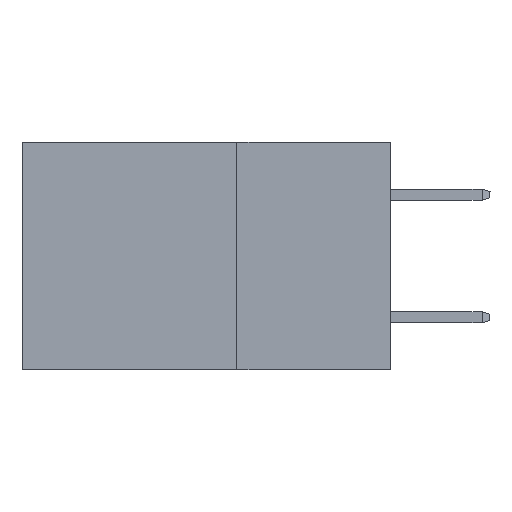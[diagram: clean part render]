
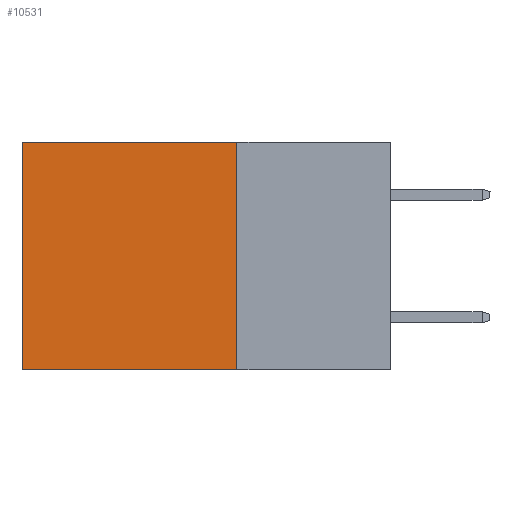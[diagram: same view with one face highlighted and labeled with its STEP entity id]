
A CAD part, left-side view. The second image highlights one B-rep face of the part: STEP entity #10531.
In plain terms, the highlighted planar face has unit normal (-1, 0, 0).
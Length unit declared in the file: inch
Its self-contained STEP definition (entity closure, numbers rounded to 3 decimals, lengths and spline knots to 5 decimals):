
#223 = DIRECTION ( 'NONE',  ( 0., 0., -1. ) ) ;
#842 = CARTESIAN_POINT ( 'NONE',  ( 0.2875, 0.25, 0. ) ) ;
#1834 = CARTESIAN_POINT ( 'NONE',  ( 0.2875, 0.25, -0.37 ) ) ;
#1917 = EDGE_CURVE ( 'NONE', #16710, #17223, #16675, .T. ) ;
#2002 = LINE ( 'NONE', #17564, #10388 ) ;
#2242 = DIRECTION ( 'NONE',  ( 1., 0., 0. ) ) ;
#2377 = VECTOR ( 'NONE', #4641, 39.37008 ) ;
#2421 = CARTESIAN_POINT ( 'NONE',  ( 0.2875, 0.25, 0. ) ) ;
#2541 = ORIENTED_EDGE ( 'NONE', *, *, #8119, .T. ) ;
#3652 = CARTESIAN_POINT ( 'NONE',  ( 0.2875, 0.25, 0. ) ) ;
#4612 = CARTESIAN_POINT ( 'NONE',  ( 0.2875, 0.6, -0.37 ) ) ;
#4641 = DIRECTION ( 'NONE',  ( 0., 1., 0. ) ) ;
#5062 = FACE_OUTER_BOUND ( 'NONE', #10837, .T. ) ;
#5237 = PLANE ( 'NONE',  #17324 ) ;
#5522 = ORIENTED_EDGE ( 'NONE', *, *, #15796, .F. ) ;
#5856 = LINE ( 'NONE', #8575, #2377 ) ;
#7149 = VERTEX_POINT ( 'NONE', #13517 ) ;
#7826 = DIRECTION ( 'NONE',  ( 0., 1., 0. ) ) ;
#8119 = EDGE_CURVE ( 'NONE', #7149, #11416, #2002, .T. ) ;
#8575 = CARTESIAN_POINT ( 'NONE',  ( 0.2875, 0.25, 0. ) ) ;
#9453 = DIRECTION ( 'NONE',  ( 0., 0., -1. ) ) ;
#10388 = VECTOR ( 'NONE', #223, 39.37008 ) ;
#10464 = CARTESIAN_POINT ( 'NONE',  ( 0.2875, 0.25, -0.37 ) ) ;
#10531 = ADVANCED_FACE ( 'NONE', ( #5062 ), #5237, .F. ) ;
#10837 = EDGE_LOOP ( 'NONE', ( #2541, #5522, #13476, #11723 ) ) ;
#11210 = EDGE_CURVE ( 'NONE', #16710, #7149, #5856, .T. ) ;
#11416 = VERTEX_POINT ( 'NONE', #4612 ) ;
#11723 = ORIENTED_EDGE ( 'NONE', *, *, #11210, .T. ) ;
#12786 = VECTOR ( 'NONE', #9453, 39.37008 ) ;
#13476 = ORIENTED_EDGE ( 'NONE', *, *, #1917, .F. ) ;
#13517 = CARTESIAN_POINT ( 'NONE',  ( 0.2875, 0.6, 0. ) ) ;
#13592 = DIRECTION ( 'NONE',  ( 0., 0., -1. ) ) ;
#15619 = VECTOR ( 'NONE', #7826, 39.37008 ) ;
#15796 = EDGE_CURVE ( 'NONE', #17223, #11416, #16260, .T. ) ;
#16260 = LINE ( 'NONE', #10464, #15619 ) ;
#16675 = LINE ( 'NONE', #842, #12786 ) ;
#16710 = VERTEX_POINT ( 'NONE', #3652 ) ;
#17223 = VERTEX_POINT ( 'NONE', #1834 ) ;
#17324 = AXIS2_PLACEMENT_3D ( 'NONE', #2421, #2242, #13592 ) ;
#17564 = CARTESIAN_POINT ( 'NONE',  ( 0.2875, 0.6, 0. ) ) ;
